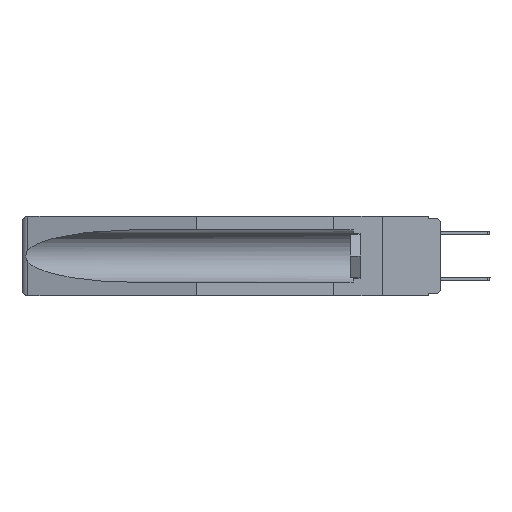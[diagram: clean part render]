
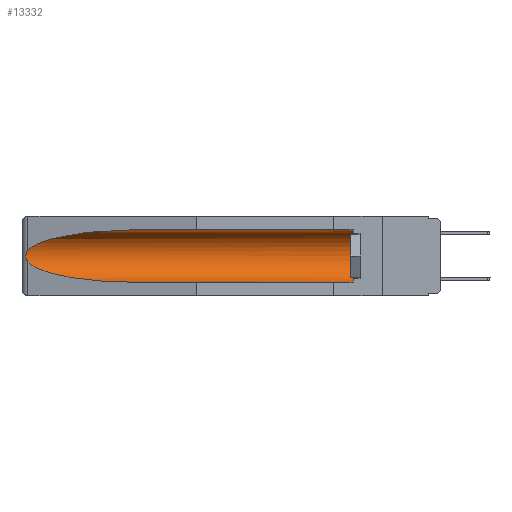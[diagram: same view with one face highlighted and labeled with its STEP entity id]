
A CAD part, left-side view. The second image highlights one B-rep face of the part: STEP entity #13332.
In plain terms, the highlighted cylindrical face has radius 2.857 mm (diameter 5.715 mm), a partial arc.
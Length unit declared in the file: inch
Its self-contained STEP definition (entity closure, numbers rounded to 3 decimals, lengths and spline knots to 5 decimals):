
#366 = VERTEX_POINT ( 'NONE', #5772 ) ;
#1217 = VERTEX_POINT ( 'NONE', #5299 ) ;
#1595 = VERTEX_POINT ( 'NONE', #16360 ) ;
#1765 = CARTESIAN_POINT ( 'NONE',  ( 0.155, -0.30754, -0.284 ) ) ;
#2163 = VERTEX_POINT ( 'NONE', #9664 ) ;
#2316 = VERTEX_POINT ( 'NONE', #11285 ) ;
#2446 =( BOUNDED_CURVE ( )  B_SPLINE_CURVE ( 3, ( #11181, #12896, #18051, #21528 ),
 .UNSPECIFIED., .F., .F. ) 
 B_SPLINE_CURVE_WITH_KNOTS ( ( 4, 4 ),
 ( 4.71239, 6.08839 ),
 .UNSPECIFIED. ) 
 CURVE ( )  GEOMETRIC_REPRESENTATION_ITEM ( )  RATIONAL_B_SPLINE_CURVE ( ( 1., 0.848, 0.848, 1. ) ) 
 REPRESENTATION_ITEM ( '' )  );
#2665 = AXIS2_PLACEMENT_3D ( 'NONE', #6090, #14795, #11149 ) ;
#2872 = ORIENTED_EDGE ( 'NONE', *, *, #18038, .T. ) ;
#2878 = LINE ( 'NONE', #1765, #15917 ) ;
#4909 = ORIENTED_EDGE ( 'NONE', *, *, #13759, .T. ) ;
#5299 = CARTESIAN_POINT ( 'NONE',  ( 0.155, 1.07973, -0.059 ) ) ;
#5344 = VERTEX_POINT ( 'NONE', #20539 ) ;
#5772 = CARTESIAN_POINT ( 'NONE',  ( 0.155, 0.126, -0.059 ) ) ;
#6090 = CARTESIAN_POINT ( 'NONE',  ( 0.155, 0.126, -0.1715 ) ) ;
#6618 = EDGE_CURVE ( 'NONE', #5344, #2163, #18333, .T. ) ;
#6633 = ORIENTED_EDGE ( 'NONE', *, *, #7934, .T. ) ;
#6753 = CARTESIAN_POINT ( 'NONE',  ( 0.2675, 1.53308, -0.16763 ) ) ;
#7934 = EDGE_CURVE ( 'NONE', #366, #1217, #15550, .T. ) ;
#8146 = VECTOR ( 'NONE', #15323, 39.37008 ) ;
#8323 = CARTESIAN_POINT ( 'NONE',  ( 0.26654, 1.53092, -0.15636 ) ) ;
#8966 = CIRCLE ( 'NONE', #2665, 0.1125 ) ;
#9035 = CARTESIAN_POINT ( 'NONE',  ( 0.21114, 1.30732, -0.284 ) ) ;
#9179 = CARTESIAN_POINT ( 'NONE',  ( 0.155, 1.07973, -0.284 ) ) ;
#9664 = CARTESIAN_POINT ( 'NONE',  ( 0.155, 1.07973, -0.284 ) ) ;
#11149 = DIRECTION ( 'NONE',  ( 0., 0., 1. ) ) ;
#11181 = CARTESIAN_POINT ( 'NONE',  ( 0.155, 1.07973, -0.059 ) ) ;
#11285 = CARTESIAN_POINT ( 'NONE',  ( 0.155, 0.126, -0.284 ) ) ;
#11721 = CARTESIAN_POINT ( 'NONE',  ( 0.2673, 1.5327, -0.16383 ) ) ;
#12679 = DIRECTION ( 'NONE',  ( 0., 1., 0. ) ) ;
#12892 = EDGE_CURVE ( 'NONE', #2316, #366, #8966, .T. ) ;
#12896 = CARTESIAN_POINT ( 'NONE',  ( 0.21114, 1.30732, -0.059 ) ) ;
#12934 = CYLINDRICAL_SURFACE ( 'NONE', #17104, 0.1125 ) ;
#13332 = ADVANCED_FACE ( 'NONE', ( #18012 ), #12934, .F. ) ;
#13387 = ORIENTED_EDGE ( 'NONE', *, *, #16870, .F. ) ;
#13579 = CARTESIAN_POINT ( 'NONE',  ( 0.26537, 1.52718, -0.19328 ) ) ;
#13759 = EDGE_CURVE ( 'NONE', #1595, #5344, #19297, .T. ) ;
#14537 = CARTESIAN_POINT ( 'NONE',  ( 0.155, -0.30754, -0.1715 ) ) ;
#14795 = DIRECTION ( 'NONE',  ( 0., -1., 0. ) ) ;
#15178 = DIRECTION ( 'NONE',  ( 0., 1., 0. ) ) ;
#15323 = DIRECTION ( 'NONE',  ( 0., 1., 0. ) ) ;
#15426 = ORIENTED_EDGE ( 'NONE', *, *, #6618, .T. ) ;
#15550 = LINE ( 'NONE', #17257, #8146 ) ;
#15917 = VECTOR ( 'NONE', #15178, 39.37008 ) ;
#16360 = CARTESIAN_POINT ( 'NONE',  ( 0.26537, 1.52718, -0.14972 ) ) ;
#16843 = CARTESIAN_POINT ( 'NONE',  ( 0.2673, 1.53269, -0.17917 ) ) ;
#16870 = EDGE_CURVE ( 'NONE', #2316, #2163, #2878, .T. ) ;
#17104 = AXIS2_PLACEMENT_3D ( 'NONE', #14537, #12679, #21176 ) ;
#17257 = CARTESIAN_POINT ( 'NONE',  ( 0.155, -0.30754, -0.059 ) ) ;
#17467 = EDGE_LOOP ( 'NONE', ( #2872, #4909, #15426, #13387, #20894, #6633 ) ) ;
#17655 = CARTESIAN_POINT ( 'NONE',  ( 0.25451, 1.48313, -0.24835 ) ) ;
#18012 = FACE_OUTER_BOUND ( 'NONE', #17467, .T. ) ;
#18038 = EDGE_CURVE ( 'NONE', #1217, #1595, #2446, .T. ) ;
#18051 = CARTESIAN_POINT ( 'NONE',  ( 0.25451, 1.48313, -0.09465 ) ) ;
#18333 =( BOUNDED_CURVE ( )  B_SPLINE_CURVE ( 3, ( #19407, #17655, #9035, #9179 ),
 .UNSPECIFIED., .F., .F. ) 
 B_SPLINE_CURVE_WITH_KNOTS ( ( 4, 4 ),
 ( 0.1948, 1.5708 ),
 .UNSPECIFIED. ) 
 CURVE ( )  GEOMETRIC_REPRESENTATION_ITEM ( )  RATIONAL_B_SPLINE_CURVE ( ( 1., 0.848, 0.848, 1. ) ) 
 REPRESENTATION_ITEM ( '' )  );
#18449 = CARTESIAN_POINT ( 'NONE',  ( 0.26597, 1.52961, -0.15275 ) ) ;
#18523 = CARTESIAN_POINT ( 'NONE',  ( 0.26537, 1.52718, -0.14972 ) ) ;
#18602 = CARTESIAN_POINT ( 'NONE',  ( 0.26597, 1.5296, -0.19026 ) ) ;
#19297 = B_SPLINE_CURVE_WITH_KNOTS ( 'NONE', 3,
 ( #18523, #18449, #8323, #11721, #6753, #20281, #16843, #21985, #18602, #13579 ),
 .UNSPECIFIED., .F., .F.,
 ( 4, 2, 2, 2, 4 ),
 ( 0., 0.00029, 0.00058, 0.00087, 0.00117 ),
 .UNSPECIFIED. ) ;
#19407 = CARTESIAN_POINT ( 'NONE',  ( 0.26537, 1.52718, -0.19328 ) ) ;
#20281 = CARTESIAN_POINT ( 'NONE',  ( 0.2675, 1.53308, -0.17534 ) ) ;
#20539 = CARTESIAN_POINT ( 'NONE',  ( 0.26537, 1.52718, -0.19328 ) ) ;
#20894 = ORIENTED_EDGE ( 'NONE', *, *, #12892, .T. ) ;
#21176 = DIRECTION ( 'NONE',  ( 0., 0., 1. ) ) ;
#21528 = CARTESIAN_POINT ( 'NONE',  ( 0.26537, 1.52718, -0.14972 ) ) ;
#21985 = CARTESIAN_POINT ( 'NONE',  ( 0.26655, 1.53094, -0.18657 ) ) ;
